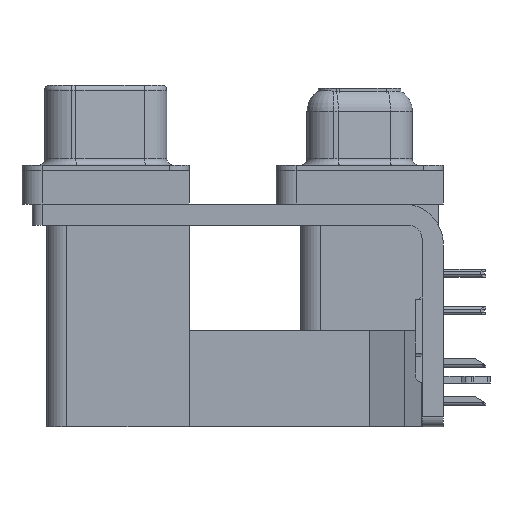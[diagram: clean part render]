
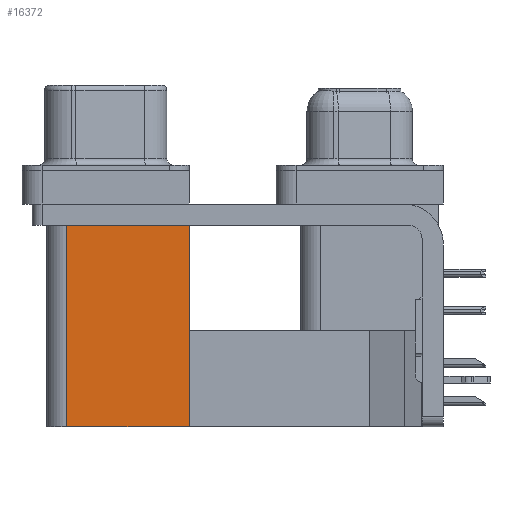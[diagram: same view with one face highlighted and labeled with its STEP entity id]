
A CAD part, left-side view. The second image highlights one B-rep face of the part: STEP entity #16372.
In plain terms, the highlighted planar face has unit normal (-1, 0, 0).
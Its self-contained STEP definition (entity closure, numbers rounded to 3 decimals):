
#1151 = DIRECTION ( 'NONE',  ( 1., 0., 0. ) ) ;
#2303 = DIRECTION ( 'NONE',  ( 0., 1., 0. ) ) ;
#2481 = LINE ( 'NONE', #30534, #32194 ) ;
#2566 = CARTESIAN_POINT ( 'NONE',  ( 3.79, 12.775, -19.2 ) ) ;
#4926 = EDGE_LOOP ( 'NONE', ( #10353, #6026, #20689, #10164 ) ) ;
#6026 = ORIENTED_EDGE ( 'NONE', *, *, #16431, .F. ) ;
#6308 = CARTESIAN_POINT ( 'NONE',  ( 3.79, 12.775, -2.5 ) ) ;
#8234 = VERTEX_POINT ( 'NONE', #6308 ) ;
#8361 = CARTESIAN_POINT ( 'NONE',  ( 3.79, 21.975, -19.2 ) ) ;
#10164 = ORIENTED_EDGE ( 'NONE', *, *, #22679, .T. ) ;
#10353 = ORIENTED_EDGE ( 'NONE', *, *, #31023, .T. ) ;
#13028 = FACE_OUTER_BOUND ( 'NONE', #4926, .T. ) ;
#16126 = DIRECTION ( 'NONE',  ( 0., 1., 0. ) ) ;
#16151 = CARTESIAN_POINT ( 'NONE',  ( 3.79, 21.975, -19.2 ) ) ;
#16372 = ADVANCED_FACE ( 'NONE', ( #13028 ), #20838, .F. ) ;
#16431 = EDGE_CURVE ( 'NONE', #29735, #27016, #30281, .T. ) ;
#18420 = DIRECTION ( 'NONE',  ( 0., 0., -1. ) ) ;
#19275 = CARTESIAN_POINT ( 'NONE',  ( 3.79, 21.975, -2.5 ) ) ;
#19298 = AXIS2_PLACEMENT_3D ( 'NONE', #24337, #1151, #18420 ) ;
#19904 = VECTOR ( 'NONE', #36212, 1000. ) ;
#20689 = ORIENTED_EDGE ( 'NONE', *, *, #26105, .F. ) ;
#20838 = PLANE ( 'NONE',  #19298 ) ;
#21881 = VECTOR ( 'NONE', #25234, 1000. ) ;
#22679 = EDGE_CURVE ( 'NONE', #22968, #8234, #25054, .T. ) ;
#22968 = VERTEX_POINT ( 'NONE', #35828 ) ;
#24337 = CARTESIAN_POINT ( 'NONE',  ( 3.79, 12.775, -19.2 ) ) ;
#25054 = LINE ( 'NONE', #28217, #21881 ) ;
#25234 = DIRECTION ( 'NONE',  ( 0., 0., 1. ) ) ;
#26105 = EDGE_CURVE ( 'NONE', #22968, #29735, #27639, .T. ) ;
#27016 = VERTEX_POINT ( 'NONE', #19275 ) ;
#27639 = LINE ( 'NONE', #2566, #30819 ) ;
#28217 = CARTESIAN_POINT ( 'NONE',  ( 3.79, 12.775, -19.2 ) ) ;
#29735 = VERTEX_POINT ( 'NONE', #8361 ) ;
#30281 = LINE ( 'NONE', #16151, #19904 ) ;
#30534 = CARTESIAN_POINT ( 'NONE',  ( 3.79, 12.775, -2.5 ) ) ;
#30819 = VECTOR ( 'NONE', #16126, 1000. ) ;
#31023 = EDGE_CURVE ( 'NONE', #8234, #27016, #2481, .T. ) ;
#32194 = VECTOR ( 'NONE', #2303, 1000. ) ;
#35828 = CARTESIAN_POINT ( 'NONE',  ( 3.79, 12.775, -19.2 ) ) ;
#36212 = DIRECTION ( 'NONE',  ( 0., 0., 1. ) ) ;
